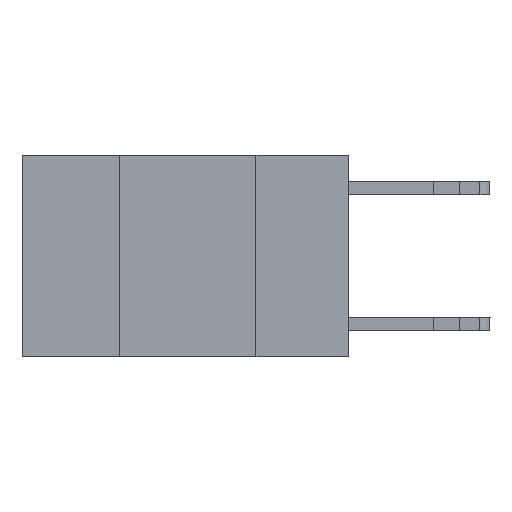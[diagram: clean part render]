
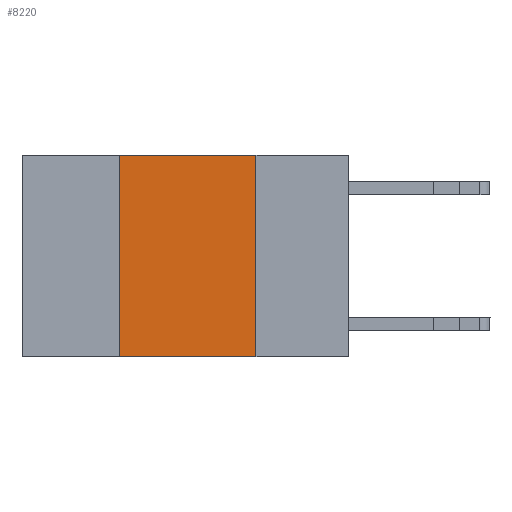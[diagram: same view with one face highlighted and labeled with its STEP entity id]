
A CAD part, left-side view. The second image highlights one B-rep face of the part: STEP entity #8220.
In plain terms, the highlighted planar face has unit normal (-1, 0, 0).
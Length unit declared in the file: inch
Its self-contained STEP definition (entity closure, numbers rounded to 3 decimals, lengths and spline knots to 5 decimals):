
#51 = ORIENTED_EDGE ( 'NONE', *, *, #466, .T. ) ;
#466 = EDGE_CURVE ( 'NONE', #4339, #10907, #11252, .T. ) ;
#1583 = EDGE_CURVE ( 'NONE', #16975, #3743, #2147, .T. ) ;
#2088 = VECTOR ( 'NONE', #18759, 39.37008 ) ;
#2147 = LINE ( 'NONE', #18730, #2088 ) ;
#3743 = VERTEX_POINT ( 'NONE', #10997 ) ;
#4339 = VERTEX_POINT ( 'NONE', #17015 ) ;
#4702 = DIRECTION ( 'NONE',  ( 0., 0., -1. ) ) ;
#4733 = DIRECTION ( 'NONE',  ( 1., 0., 0. ) ) ;
#4809 = CARTESIAN_POINT ( 'NONE',  ( 0., 0.6, 0. ) ) ;
#4840 = PLANE ( 'NONE',  #7885 ) ;
#5468 = DIRECTION ( 'NONE',  ( 0., -1., 0. ) ) ;
#5476 = CARTESIAN_POINT ( 'NONE',  ( 0., 0.6, -0.37 ) ) ;
#7885 = AXIS2_PLACEMENT_3D ( 'NONE', #4809, #4733, #4702 ) ;
#8220 = ADVANCED_FACE ( 'NONE', ( #17493 ), #4840, .F. ) ;
#9253 = VECTOR ( 'NONE', #13763, 39.37008 ) ;
#10907 = VERTEX_POINT ( 'NONE', #22339 ) ;
#10997 = CARTESIAN_POINT ( 'NONE',  ( 0., 0.17, 0. ) ) ;
#11234 = LINE ( 'NONE', #17262, #9253 ) ;
#11250 = EDGE_CURVE ( 'NONE', #3743, #10907, #19535, .T. ) ;
#11252 = LINE ( 'NONE', #5476, #11360 ) ;
#11360 = VECTOR ( 'NONE', #5468, 39.37008 ) ;
#13192 = EDGE_LOOP ( 'NONE', ( #22756, #23005, #23247, #51 ) ) ;
#13763 = DIRECTION ( 'NONE',  ( 0., 0., 1. ) ) ;
#14691 = CARTESIAN_POINT ( 'NONE',  ( 0., 0.42, 0. ) ) ;
#16975 = VERTEX_POINT ( 'NONE', #14691 ) ;
#17015 = CARTESIAN_POINT ( 'NONE',  ( 0., 0.42, -0.37 ) ) ;
#17262 = CARTESIAN_POINT ( 'NONE',  ( 0., 0.42, 0. ) ) ;
#17331 = CARTESIAN_POINT ( 'NONE',  ( 0., 0.17, 0. ) ) ;
#17404 = DIRECTION ( 'NONE',  ( 0., 0., -1. ) ) ;
#17493 = FACE_OUTER_BOUND ( 'NONE', #13192, .T. ) ;
#18730 = CARTESIAN_POINT ( 'NONE',  ( 0., 0.6, 0. ) ) ;
#18759 = DIRECTION ( 'NONE',  ( 0., -1., 0. ) ) ;
#19293 = EDGE_CURVE ( 'NONE', #4339, #16975, #11234, .T. ) ;
#19535 = LINE ( 'NONE', #17331, #19811 ) ;
#19811 = VECTOR ( 'NONE', #17404, 39.37008 ) ;
#22339 = CARTESIAN_POINT ( 'NONE',  ( 0., 0.17, -0.37 ) ) ;
#22756 = ORIENTED_EDGE ( 'NONE', *, *, #11250, .F. ) ;
#23005 = ORIENTED_EDGE ( 'NONE', *, *, #1583, .F. ) ;
#23247 = ORIENTED_EDGE ( 'NONE', *, *, #19293, .F. ) ;
